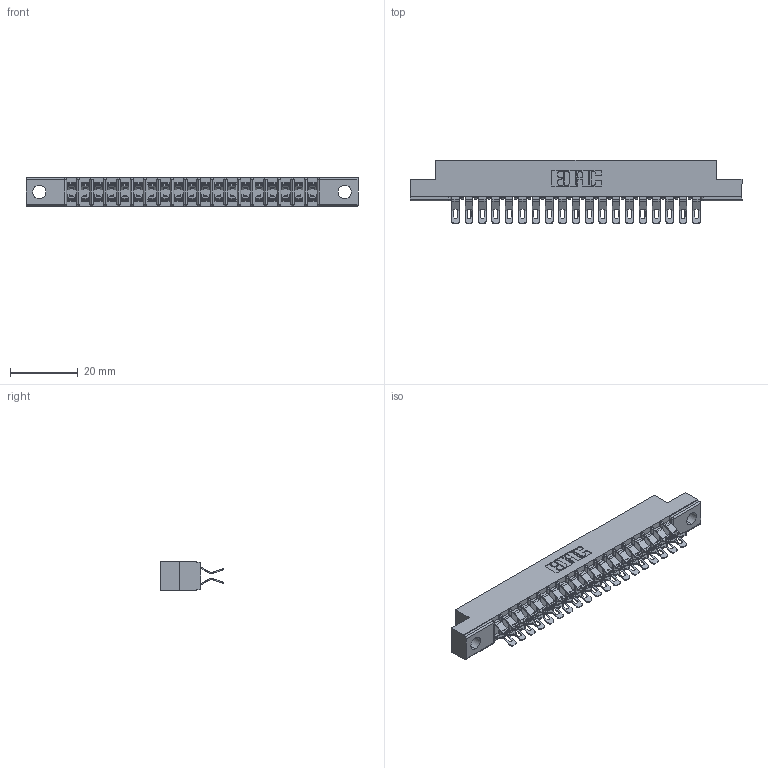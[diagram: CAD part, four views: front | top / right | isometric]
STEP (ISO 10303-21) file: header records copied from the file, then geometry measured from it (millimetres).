
FILE_DESCRIPTION (( 'STEP AP203' ), '1' );
FILE_NAME ('357-038-555-202.STEP', '2018-08-10T10:08:39', ( '' ), ( '' ), 'SwSTEP 2.0', 'SolidWorks 2016', '' );
FILE_SCHEMA (( 'CONFIG_CONTROL_DESIGN' ));
Length unit declared in the file: inch
Products named in the file (3): 307 Part_.128 Dia Mounting Holes; 307-290-001_555; 357-038-555-202
Assembly tree (39 placements, depth 2):
  357-038-555-202
    307 Part_.128 Dia Mounting Holes
    307-290-001_555  x38
Bounding box: 98.3 x 18.75 x 8.71 mm (x, y, z)
Volume: 6455.4 mm3; surface area: 11717.6 mm2
Topology: 39 solids, 39 shells, 2456 faces, 7201 edges, 4694 vertices
Faces by surface type: plane 1362, cylinder 1054, sphere 40
Entity records: 20271 total; most frequent: CARTESIAN_POINT 3327, ORIENTED_EDGE 3296, DIRECTION 3276, EDGE_CURVE 1648, LINE 1242, VECTOR 1242, VERTEX_POINT 1068, AXIS2_PLACEMENT_3D 1017
